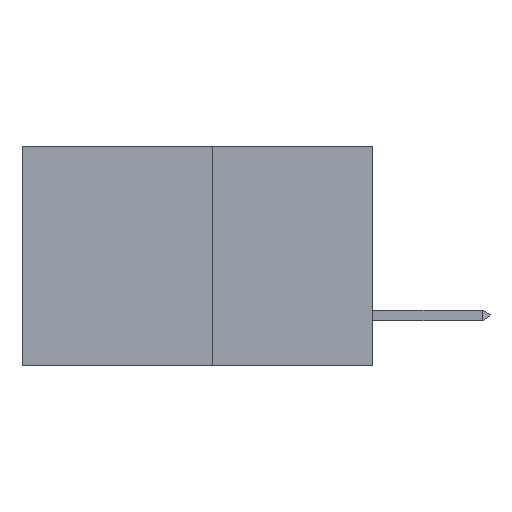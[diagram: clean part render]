
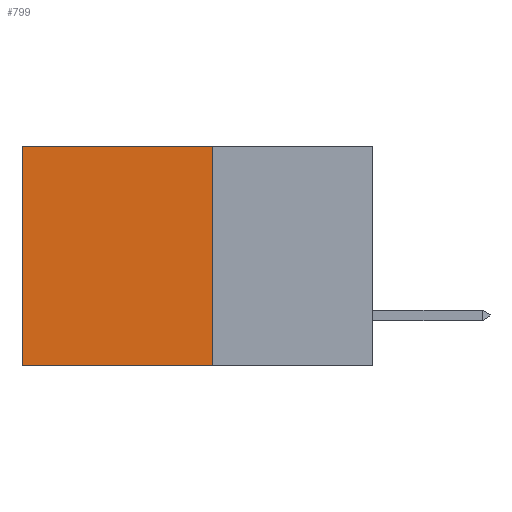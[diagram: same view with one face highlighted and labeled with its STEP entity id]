
A CAD part, left-side view. The second image highlights one B-rep face of the part: STEP entity #799.
In plain terms, the highlighted planar face has unit normal (-1, 0, 0).
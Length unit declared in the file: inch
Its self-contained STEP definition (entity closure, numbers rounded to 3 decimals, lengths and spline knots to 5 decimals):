
#176 = EDGE_CURVE ( 'NONE', #12992, #2471, #15099, .T. ) ;
#272 = VERTEX_POINT ( 'NONE', #11603 ) ;
#724 = CARTESIAN_POINT ( 'NONE',  ( 0.277, 0.27, -0.37 ) ) ;
#799 = ADVANCED_FACE ( 'NONE', ( #5626 ), #7836, .F. ) ;
#1695 = VECTOR ( 'NONE', #2102, 39.37008 ) ;
#1738 = CARTESIAN_POINT ( 'NONE',  ( 0.277, 0.27, -0.37 ) ) ;
#2102 = DIRECTION ( 'NONE',  ( 0., 0., -1. ) ) ;
#2471 = VERTEX_POINT ( 'NONE', #13116 ) ;
#3134 = ORIENTED_EDGE ( 'NONE', *, *, #10575, .F. ) ;
#3862 = DIRECTION ( 'NONE',  ( 0., 0., -1. ) ) ;
#5106 = VECTOR ( 'NONE', #9724, 39.37008 ) ;
#5299 = ORIENTED_EDGE ( 'NONE', *, *, #176, .F. ) ;
#5626 = FACE_OUTER_BOUND ( 'NONE', #16189, .T. ) ;
#5704 = CARTESIAN_POINT ( 'NONE',  ( 0.277, 0.27, 0. ) ) ;
#6269 = DIRECTION ( 'NONE',  ( 0., 1., 0. ) ) ;
#6627 = DIRECTION ( 'NONE',  ( 0., 0., -1. ) ) ;
#7776 = EDGE_CURVE ( 'NONE', #272, #2471, #16110, .T. ) ;
#7836 = PLANE ( 'NONE',  #13191 ) ;
#8391 = LINE ( 'NONE', #724, #1695 ) ;
#8647 = VERTEX_POINT ( 'NONE', #5704 ) ;
#9724 = DIRECTION ( 'NONE',  ( 0., 1., 0. ) ) ;
#10015 = ORIENTED_EDGE ( 'NONE', *, *, #7776, .T. ) ;
#10345 = CARTESIAN_POINT ( 'NONE',  ( 0.277, 0.27, -0.37 ) ) ;
#10575 = EDGE_CURVE ( 'NONE', #8647, #12992, #8391, .T. ) ;
#10919 = CARTESIAN_POINT ( 'NONE',  ( 0.277, 0.27, 0. ) ) ;
#11053 = VECTOR ( 'NONE', #6269, 39.37008 ) ;
#11603 = CARTESIAN_POINT ( 'NONE',  ( 0.277, 0.59, 0. ) ) ;
#12211 = DIRECTION ( 'NONE',  ( 1., 0., 0. ) ) ;
#12703 = CARTESIAN_POINT ( 'NONE',  ( 0.277, 0.59, -0.37 ) ) ;
#12824 = VECTOR ( 'NONE', #6627, 39.37008 ) ;
#12992 = VERTEX_POINT ( 'NONE', #1738 ) ;
#13116 = CARTESIAN_POINT ( 'NONE',  ( 0.277, 0.59, -0.37 ) ) ;
#13191 = AXIS2_PLACEMENT_3D ( 'NONE', #13688, #12211, #3862 ) ;
#13688 = CARTESIAN_POINT ( 'NONE',  ( 0.277, 0.27, -0.37 ) ) ;
#14868 = ORIENTED_EDGE ( 'NONE', *, *, #15665, .T. ) ;
#14966 = LINE ( 'NONE', #10919, #5106 ) ;
#15099 = LINE ( 'NONE', #10345, #11053 ) ;
#15665 = EDGE_CURVE ( 'NONE', #8647, #272, #14966, .T. ) ;
#16110 = LINE ( 'NONE', #12703, #12824 ) ;
#16189 = EDGE_LOOP ( 'NONE', ( #10015, #5299, #3134, #14868 ) ) ;
